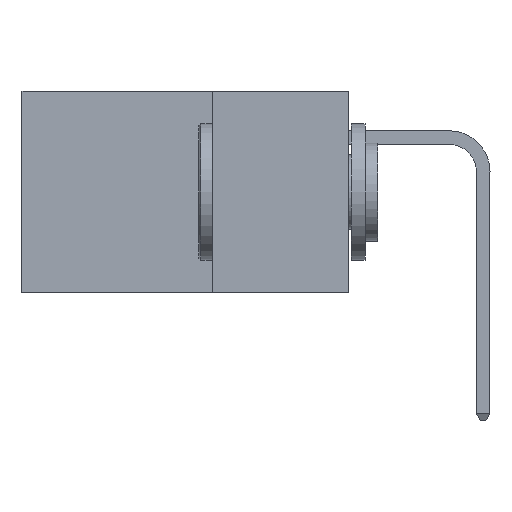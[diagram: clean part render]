
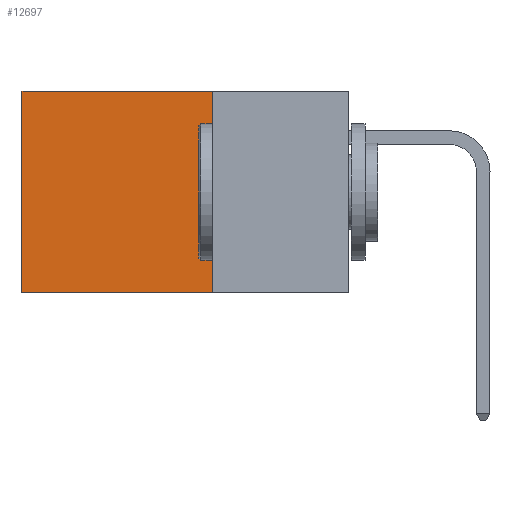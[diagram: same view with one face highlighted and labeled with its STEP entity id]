
A CAD part, left-side view. The second image highlights one B-rep face of the part: STEP entity #12697.
In plain terms, the highlighted planar face has unit normal (-1, 0, 0).
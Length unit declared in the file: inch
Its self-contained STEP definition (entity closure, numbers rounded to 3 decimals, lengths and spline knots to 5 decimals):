
#521 = LINE ( 'NONE', #13905, #10165 ) ;
#1318 = DIRECTION ( 'NONE',  ( 0., 0., -1. ) ) ;
#1986 = LINE ( 'NONE', #8090, #4961 ) ;
#3012 = ORIENTED_EDGE ( 'NONE', *, *, #4966, .T. ) ;
#3158 = PLANE ( 'NONE',  #7866 ) ;
#3595 = LINE ( 'NONE', #7248, #9863 ) ;
#4239 = CARTESIAN_POINT ( 'NONE',  ( 0.2875, 0.6, 0. ) ) ;
#4845 = CARTESIAN_POINT ( 'NONE',  ( 0.2875, 0.25, 0. ) ) ;
#4961 = VECTOR ( 'NONE', #6826, 39.37008 ) ;
#4966 = EDGE_CURVE ( 'NONE', #13947, #15608, #3595, .T. ) ;
#5075 = LINE ( 'NONE', #10436, #14665 ) ;
#5708 = DIRECTION ( 'NONE',  ( 0., 0., -1. ) ) ;
#6075 = CARTESIAN_POINT ( 'NONE',  ( 0.2875, 0.25, -0.37 ) ) ;
#6576 = ORIENTED_EDGE ( 'NONE', *, *, #8984, .F. ) ;
#6826 = DIRECTION ( 'NONE',  ( 0., 0., -1. ) ) ;
#7056 = EDGE_CURVE ( 'NONE', #15608, #14709, #521, .T. ) ;
#7248 = CARTESIAN_POINT ( 'NONE',  ( 0.2875, 0.25, 0. ) ) ;
#7866 = AXIS2_PLACEMENT_3D ( 'NONE', #11925, #13194, #5708 ) ;
#8015 = ORIENTED_EDGE ( 'NONE', *, *, #13188, .F. ) ;
#8090 = CARTESIAN_POINT ( 'NONE',  ( 0.2875, 0.25, 0. ) ) ;
#8491 = ORIENTED_EDGE ( 'NONE', *, *, #7056, .T. ) ;
#8984 = EDGE_CURVE ( 'NONE', #15925, #14709, #5075, .T. ) ;
#9863 = VECTOR ( 'NONE', #14767, 39.37008 ) ;
#10165 = VECTOR ( 'NONE', #1318, 39.37008 ) ;
#10436 = CARTESIAN_POINT ( 'NONE',  ( 0.2875, 0.25, -0.37 ) ) ;
#11677 = DIRECTION ( 'NONE',  ( 0., 1., 0. ) ) ;
#11925 = CARTESIAN_POINT ( 'NONE',  ( 0.2875, 0.25, 0. ) ) ;
#12380 = FACE_OUTER_BOUND ( 'NONE', #13675, .T. ) ;
#12697 = ADVANCED_FACE ( 'NONE', ( #12380 ), #3158, .F. ) ;
#13188 = EDGE_CURVE ( 'NONE', #13947, #15925, #1986, .T. ) ;
#13194 = DIRECTION ( 'NONE',  ( 1., 0., 0. ) ) ;
#13675 = EDGE_LOOP ( 'NONE', ( #8491, #6576, #8015, #3012 ) ) ;
#13905 = CARTESIAN_POINT ( 'NONE',  ( 0.2875, 0.6, 0. ) ) ;
#13947 = VERTEX_POINT ( 'NONE', #4845 ) ;
#14665 = VECTOR ( 'NONE', #11677, 39.37008 ) ;
#14709 = VERTEX_POINT ( 'NONE', #14996 ) ;
#14767 = DIRECTION ( 'NONE',  ( 0., 1., 0. ) ) ;
#14996 = CARTESIAN_POINT ( 'NONE',  ( 0.2875, 0.6, -0.37 ) ) ;
#15608 = VERTEX_POINT ( 'NONE', #4239 ) ;
#15925 = VERTEX_POINT ( 'NONE', #6075 ) ;
